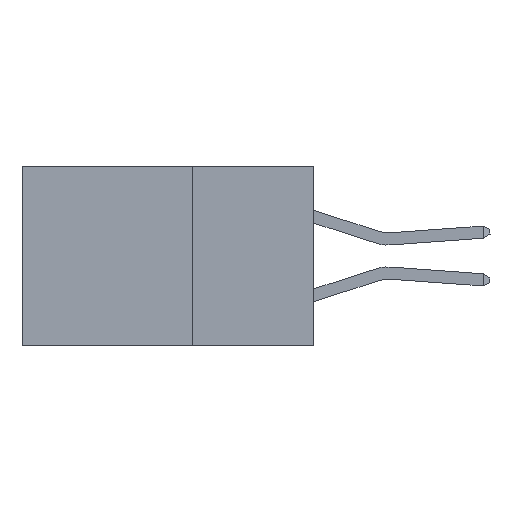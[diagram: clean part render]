
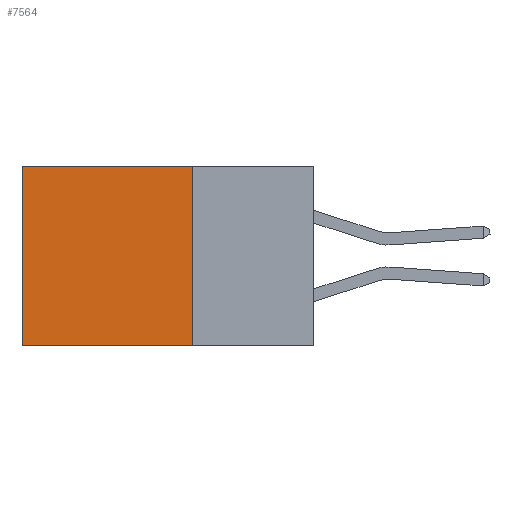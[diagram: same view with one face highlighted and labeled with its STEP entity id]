
A CAD part, left-side view. The second image highlights one B-rep face of the part: STEP entity #7564.
In plain terms, the highlighted planar face has unit normal (-1, 0, 0).
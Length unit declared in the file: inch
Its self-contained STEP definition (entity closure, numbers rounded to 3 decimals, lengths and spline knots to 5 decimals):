
#555 = ORIENTED_EDGE ( 'NONE', *, *, #12318, .T. ) ;
#822 = DIRECTION ( 'NONE',  ( 0., 0., -1. ) ) ;
#1199 = LINE ( 'NONE', #14600, #17353 ) ;
#2080 = DIRECTION ( 'NONE',  ( 1., 0., 0. ) ) ;
#2226 = EDGE_CURVE ( 'NONE', #18990, #2665, #15763, .T. ) ;
#2569 = ORIENTED_EDGE ( 'NONE', *, *, #2978, .F. ) ;
#2665 = VERTEX_POINT ( 'NONE', #3607 ) ;
#2978 = EDGE_CURVE ( 'NONE', #6059, #2665, #14970, .T. ) ;
#3607 = CARTESIAN_POINT ( 'NONE',  ( 0.2875, 0.6, -0.37 ) ) ;
#3631 = DIRECTION ( 'NONE',  ( 0., 0., -1. ) ) ;
#3654 = LINE ( 'NONE', #15413, #16779 ) ;
#4046 = CARTESIAN_POINT ( 'NONE',  ( 0.2875, 0.25, -0.37 ) ) ;
#4389 = VECTOR ( 'NONE', #822, 39.37008 ) ;
#5737 = CARTESIAN_POINT ( 'NONE',  ( 0.2875, 0.6, 0. ) ) ;
#6059 = VERTEX_POINT ( 'NONE', #9865 ) ;
#6708 = FACE_OUTER_BOUND ( 'NONE', #17429, .T. ) ;
#6772 = ORIENTED_EDGE ( 'NONE', *, *, #18965, .F. ) ;
#7564 = ADVANCED_FACE ( 'NONE', ( #6708 ), #8182, .F. ) ;
#8182 = PLANE ( 'NONE',  #12340 ) ;
#9546 = CARTESIAN_POINT ( 'NONE',  ( 0.2875, 0.25, 0. ) ) ;
#9750 = ORIENTED_EDGE ( 'NONE', *, *, #2226, .T. ) ;
#9865 = CARTESIAN_POINT ( 'NONE',  ( 0.2875, 0.25, -0.37 ) ) ;
#10026 = DIRECTION ( 'NONE',  ( 0., 0., -1. ) ) ;
#10405 = VERTEX_POINT ( 'NONE', #15285 ) ;
#11136 = DIRECTION ( 'NONE',  ( 0., 1., 0. ) ) ;
#12318 = EDGE_CURVE ( 'NONE', #10405, #18990, #3654, .T. ) ;
#12340 = AXIS2_PLACEMENT_3D ( 'NONE', #9546, #2080, #3631 ) ;
#13918 = VECTOR ( 'NONE', #16290, 39.37008 ) ;
#14600 = CARTESIAN_POINT ( 'NONE',  ( 0.2875, 0.25, 0. ) ) ;
#14970 = LINE ( 'NONE', #4046, #13918 ) ;
#15285 = CARTESIAN_POINT ( 'NONE',  ( 0.2875, 0.25, 0. ) ) ;
#15413 = CARTESIAN_POINT ( 'NONE',  ( 0.2875, 0.25, 0. ) ) ;
#15673 = CARTESIAN_POINT ( 'NONE',  ( 0.2875, 0.6, 0. ) ) ;
#15763 = LINE ( 'NONE', #15673, #4389 ) ;
#16290 = DIRECTION ( 'NONE',  ( 0., 1., 0. ) ) ;
#16779 = VECTOR ( 'NONE', #11136, 39.37008 ) ;
#17353 = VECTOR ( 'NONE', #10026, 39.37008 ) ;
#17429 = EDGE_LOOP ( 'NONE', ( #9750, #2569, #6772, #555 ) ) ;
#18965 = EDGE_CURVE ( 'NONE', #10405, #6059, #1199, .T. ) ;
#18990 = VERTEX_POINT ( 'NONE', #5737 ) ;
